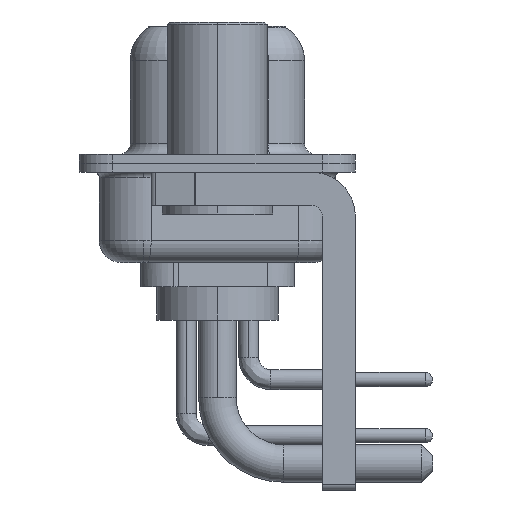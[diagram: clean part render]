
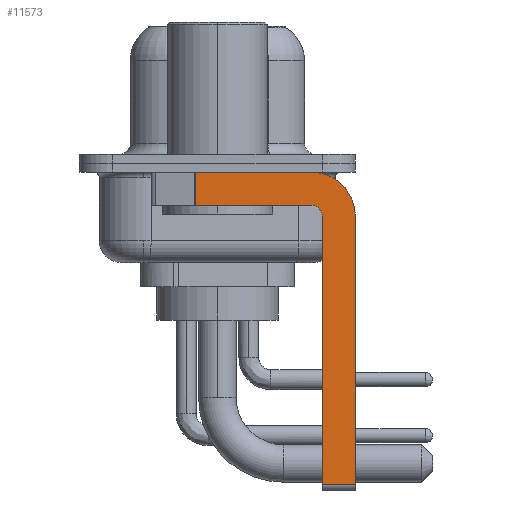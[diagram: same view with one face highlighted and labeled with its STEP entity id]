
A CAD part, left-side view. The second image highlights one B-rep face of the part: STEP entity #11573.
In plain terms, the highlighted planar face has unit normal (-1, 0, 0).
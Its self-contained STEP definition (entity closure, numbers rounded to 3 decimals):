
#5 = EDGE_CURVE ( 'NONE', #22372, #8908, #1338, .T. ) ;
#712 = VERTEX_POINT ( 'NONE', #9219 ) ;
#1006 = VERTEX_POINT ( 'NONE', #11951 ) ;
#1338 = CIRCLE ( 'NONE', #7241, 2. ) ;
#1392 = CARTESIAN_POINT ( 'NONE',  ( -2.9, -4.75, -2.4 ) ) ;
#1474 = VERTEX_POINT ( 'NONE', #1392 ) ;
#1617 = EDGE_CURVE ( 'NONE', #9940, #22372, #7270, .T. ) ;
#1941 = DIRECTION ( 'NONE',  ( 0., 0., 1. ) ) ;
#2137 = CARTESIAN_POINT ( 'NONE',  ( -2.9, -6.25, -2.4 ) ) ;
#2587 = CARTESIAN_POINT ( 'NONE',  ( -2.9, -6.25, -14.55 ) ) ;
#3338 = LINE ( 'NONE', #18989, #18225 ) ;
#3609 = LINE ( 'NONE', #21105, #11972 ) ;
#4008 = LINE ( 'NONE', #11033, #22598 ) ;
#4198 = VECTOR ( 'NONE', #1941, 1000. ) ;
#4669 = EDGE_CURVE ( 'NONE', #1474, #712, #15551, .T. ) ;
#5301 = LINE ( 'NONE', #10718, #4198 ) ;
#5919 = CARTESIAN_POINT ( 'NONE',  ( -2.9, 0.978, -1.9 ) ) ;
#6168 = CARTESIAN_POINT ( 'NONE',  ( -2.9, -4.25, -0.4 ) ) ;
#6339 = ORIENTED_EDGE ( 'NONE', *, *, #4669, .F. ) ;
#6486 = VERTEX_POINT ( 'NONE', #9367 ) ;
#6824 = EDGE_CURVE ( 'NONE', #1006, #1474, #5301, .T. ) ;
#7241 = AXIS2_PLACEMENT_3D ( 'NONE', #16844, #21670, #16505 ) ;
#7270 = LINE ( 'NONE', #21388, #21280 ) ;
#7297 = CARTESIAN_POINT ( 'NONE',  ( -2.9, -4.25, -2.4 ) ) ;
#7588 = EDGE_CURVE ( 'NONE', #9940, #6486, #11557, .T. ) ;
#7626 = DIRECTION ( 'NONE',  ( 1., 0., 0. ) ) ;
#7889 = CARTESIAN_POINT ( 'NONE',  ( -2.9, 0.978, -0.4 ) ) ;
#8355 = DIRECTION ( 'NONE',  ( 0., 0., -1. ) ) ;
#8881 = DIRECTION ( 'NONE',  ( 0., 1., 0. ) ) ;
#8908 = VERTEX_POINT ( 'NONE', #2137 ) ;
#9181 = ORIENTED_EDGE ( 'NONE', *, *, #20275, .F. ) ;
#9219 = CARTESIAN_POINT ( 'NONE',  ( -2.9, -4.25, -1.9 ) ) ;
#9221 = DIRECTION ( 'NONE',  ( 0., -1., 0. ) ) ;
#9365 = DIRECTION ( 'NONE',  ( 0., 0., -1. ) ) ;
#9367 = CARTESIAN_POINT ( 'NONE',  ( -2.9, 0.978, -1.9 ) ) ;
#9940 = VERTEX_POINT ( 'NONE', #7889 ) ;
#10718 = CARTESIAN_POINT ( 'NONE',  ( -2.9, -4.75, -14.8 ) ) ;
#10741 = ORIENTED_EDGE ( 'NONE', *, *, #13693, .F. ) ;
#11033 = CARTESIAN_POINT ( 'NONE',  ( -2.9, -4.25, -1.9 ) ) ;
#11150 = AXIS2_PLACEMENT_3D ( 'NONE', #7297, #7626, #9365 ) ;
#11257 = DIRECTION ( 'NONE',  ( -1., 0., 0. ) ) ;
#11374 = DIRECTION ( 'NONE',  ( 0., 0., 1. ) ) ;
#11550 = ORIENTED_EDGE ( 'NONE', *, *, #1617, .F. ) ;
#11557 = LINE ( 'NONE', #5919, #18282 ) ;
#11573 = ADVANCED_FACE ( 'NONE', ( #17978 ), #21638, .F. ) ;
#11951 = CARTESIAN_POINT ( 'NONE',  ( -2.9, -4.75, -14.55 ) ) ;
#11972 = VECTOR ( 'NONE', #21212, 1000. ) ;
#12536 = ORIENTED_EDGE ( 'NONE', *, *, #5, .F. ) ;
#13693 = EDGE_CURVE ( 'NONE', #8908, #16089, #3609, .T. ) ;
#13704 = AXIS2_PLACEMENT_3D ( 'NONE', #20012, #11257, #11374 ) ;
#13764 = ORIENTED_EDGE ( 'NONE', *, *, #6824, .F. ) ;
#14099 = EDGE_CURVE ( 'NONE', #1006, #16089, #3338, .T. ) ;
#15551 = CIRCLE ( 'NONE', #13704, 0.5 ) ;
#16089 = VERTEX_POINT ( 'NONE', #2587 ) ;
#16505 = DIRECTION ( 'NONE',  ( 0., 0., -1. ) ) ;
#16594 = DIRECTION ( 'NONE',  ( 0., -1., 0. ) ) ;
#16844 = CARTESIAN_POINT ( 'NONE',  ( -2.9, -4.25, -2.4 ) ) ;
#17891 = EDGE_LOOP ( 'NONE', ( #11550, #19262, #9181, #6339, #13764, #22406, #10741, #12536 ) ) ;
#17978 = FACE_OUTER_BOUND ( 'NONE', #17891, .T. ) ;
#18225 = VECTOR ( 'NONE', #16594, 1000. ) ;
#18282 = VECTOR ( 'NONE', #8355, 1000. ) ;
#18989 = CARTESIAN_POINT ( 'NONE',  ( -2.9, -4.25, -14.55 ) ) ;
#19262 = ORIENTED_EDGE ( 'NONE', *, *, #7588, .T. ) ;
#20012 = CARTESIAN_POINT ( 'NONE',  ( -2.9, -4.25, -2.4 ) ) ;
#20275 = EDGE_CURVE ( 'NONE', #712, #6486, #4008, .T. ) ;
#21105 = CARTESIAN_POINT ( 'NONE',  ( -2.9, -6.25, -2.4 ) ) ;
#21212 = DIRECTION ( 'NONE',  ( 0., 0., -1. ) ) ;
#21280 = VECTOR ( 'NONE', #9221, 1000. ) ;
#21388 = CARTESIAN_POINT ( 'NONE',  ( -2.9, 3., -0.4 ) ) ;
#21638 = PLANE ( 'NONE',  #11150 ) ;
#21670 = DIRECTION ( 'NONE',  ( 1., 0., 0. ) ) ;
#22372 = VERTEX_POINT ( 'NONE', #6168 ) ;
#22406 = ORIENTED_EDGE ( 'NONE', *, *, #14099, .T. ) ;
#22598 = VECTOR ( 'NONE', #8881, 1000. ) ;
